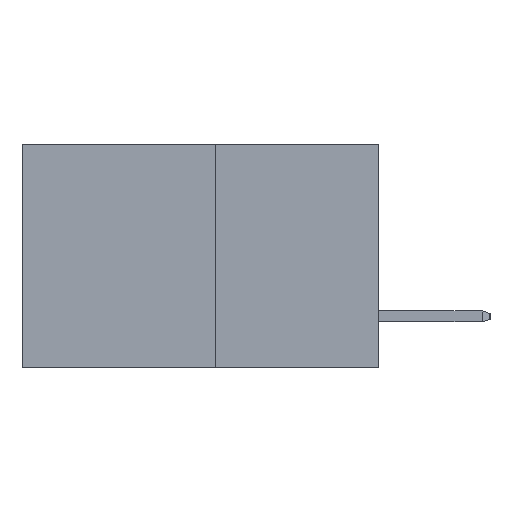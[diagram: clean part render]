
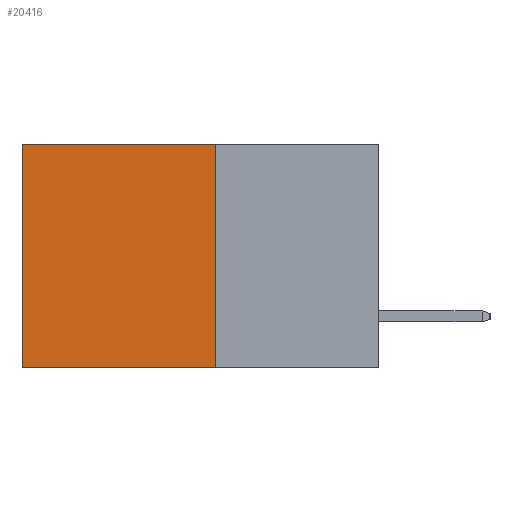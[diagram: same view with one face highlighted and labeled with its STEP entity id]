
A CAD part, left-side view. The second image highlights one B-rep face of the part: STEP entity #20416.
In plain terms, the highlighted planar face has unit normal (-1, 0, 0).
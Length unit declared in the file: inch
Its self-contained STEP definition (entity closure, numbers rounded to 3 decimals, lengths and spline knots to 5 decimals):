
#390 = ORIENTED_EDGE ( 'NONE', *, *, #11512, .F. ) ;
#1002 = CARTESIAN_POINT ( 'NONE',  ( 0.277, 0.27, -0.37 ) ) ;
#1298 = CARTESIAN_POINT ( 'NONE',  ( 0.277, 0.27, -0.37 ) ) ;
#1336 = VERTEX_POINT ( 'NONE', #12384 ) ;
#2784 = EDGE_CURVE ( 'NONE', #9355, #27228, #15177, .T. ) ;
#3221 = DIRECTION ( 'NONE',  ( 0., 0., -1. ) ) ;
#3382 = DIRECTION ( 'NONE',  ( 0., 0., -1. ) ) ;
#6019 = CARTESIAN_POINT ( 'NONE',  ( 0.277, 0.59, -0.37 ) ) ;
#6435 = VECTOR ( 'NONE', #14427, 39.37008 ) ;
#6884 = CARTESIAN_POINT ( 'NONE',  ( 0.277, 0.59, 0. ) ) ;
#8496 = DIRECTION ( 'NONE',  ( 0., 1., 0. ) ) ;
#9355 = VERTEX_POINT ( 'NONE', #6884 ) ;
#9732 = PLANE ( 'NONE',  #25160 ) ;
#10975 = ORIENTED_EDGE ( 'NONE', *, *, #12802, .F. ) ;
#11512 = EDGE_CURVE ( 'NONE', #12450, #27228, #23535, .T. ) ;
#11515 = VECTOR ( 'NONE', #8496, 39.37008 ) ;
#11958 = VECTOR ( 'NONE', #24992, 39.37008 ) ;
#12193 = LINE ( 'NONE', #21646, #11515 ) ;
#12384 = CARTESIAN_POINT ( 'NONE',  ( 0.277, 0.27, 0. ) ) ;
#12450 = VERTEX_POINT ( 'NONE', #24131 ) ;
#12802 = EDGE_CURVE ( 'NONE', #1336, #12450, #23843, .T. ) ;
#14421 = CARTESIAN_POINT ( 'NONE',  ( 0.277, 0.59, -0.37 ) ) ;
#14427 = DIRECTION ( 'NONE',  ( 0., 0., -1. ) ) ;
#15177 = LINE ( 'NONE', #6019, #20270 ) ;
#16331 = DIRECTION ( 'NONE',  ( 1., 0., 0. ) ) ;
#20270 = VECTOR ( 'NONE', #3382, 39.37008 ) ;
#20416 = ADVANCED_FACE ( 'NONE', ( #27520 ), #9732, .F. ) ;
#20961 = EDGE_LOOP ( 'NONE', ( #24640, #390, #10975, #21673 ) ) ;
#21646 = CARTESIAN_POINT ( 'NONE',  ( 0.277, 0.27, 0. ) ) ;
#21673 = ORIENTED_EDGE ( 'NONE', *, *, #22667, .T. ) ;
#22667 = EDGE_CURVE ( 'NONE', #1336, #9355, #12193, .T. ) ;
#22829 = CARTESIAN_POINT ( 'NONE',  ( 0.277, 0.27, -0.37 ) ) ;
#23535 = LINE ( 'NONE', #22829, #11958 ) ;
#23843 = LINE ( 'NONE', #1298, #6435 ) ;
#24131 = CARTESIAN_POINT ( 'NONE',  ( 0.277, 0.27, -0.37 ) ) ;
#24640 = ORIENTED_EDGE ( 'NONE', *, *, #2784, .T. ) ;
#24992 = DIRECTION ( 'NONE',  ( 0., 1., 0. ) ) ;
#25160 = AXIS2_PLACEMENT_3D ( 'NONE', #1002, #16331, #3221 ) ;
#27228 = VERTEX_POINT ( 'NONE', #14421 ) ;
#27520 = FACE_OUTER_BOUND ( 'NONE', #20961, .T. ) ;
